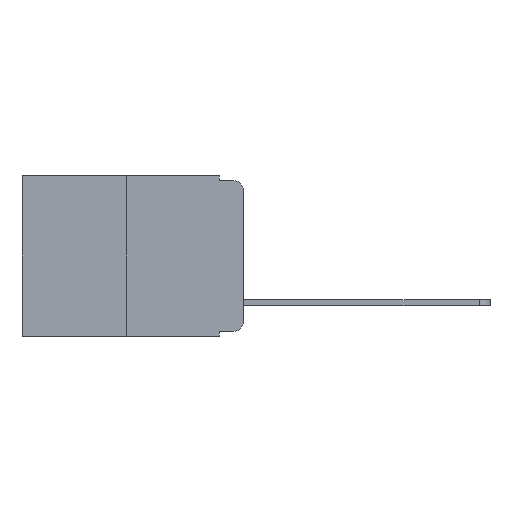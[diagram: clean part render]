
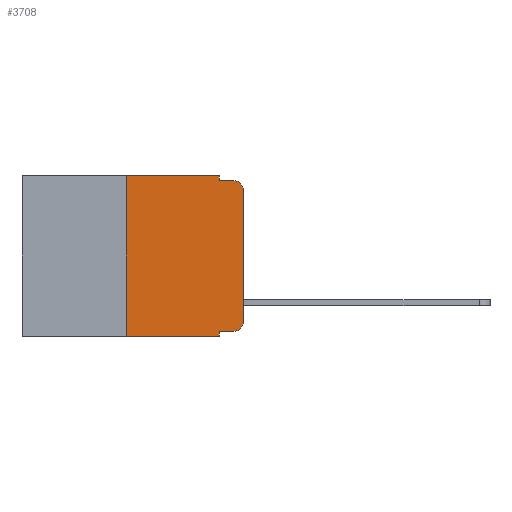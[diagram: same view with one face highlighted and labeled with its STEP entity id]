
A CAD part, left-side view. The second image highlights one B-rep face of the part: STEP entity #3708.
In plain terms, the highlighted planar face has unit normal (-1, 0, 0).
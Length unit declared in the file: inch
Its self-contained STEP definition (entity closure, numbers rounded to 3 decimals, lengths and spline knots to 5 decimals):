
#467 = ORIENTED_EDGE ( 'NONE', *, *, #6328, .F. ) ;
#604 = VERTEX_POINT ( 'NONE', #6772 ) ;
#728 = VERTEX_POINT ( 'NONE', #13608 ) ;
#889 = AXIS2_PLACEMENT_3D ( 'NONE', #8602, #965, #9829 ) ;
#965 = DIRECTION ( 'NONE',  ( -1., 0., 0. ) ) ;
#1081 = EDGE_CURVE ( 'NONE', #11808, #11613, #7560, .T. ) ;
#1479 = CARTESIAN_POINT ( 'NONE',  ( 0., 0.051, -0.01 ) ) ;
#1660 = EDGE_CURVE ( 'NONE', #11613, #728, #3568, .T. ) ;
#1695 = ORIENTED_EDGE ( 'NONE', *, *, #7569, .T. ) ;
#1840 = VERTEX_POINT ( 'NONE', #5149 ) ;
#2181 = CARTESIAN_POINT ( 'NONE',  ( 0., 0., -0.03 ) ) ;
#2254 = CARTESIAN_POINT ( 'NONE',  ( 0., 0.25, -0.343 ) ) ;
#2334 = VERTEX_POINT ( 'NONE', #11303 ) ;
#3093 = DIRECTION ( 'NONE',  ( 0., 0., -1. ) ) ;
#3274 = EDGE_CURVE ( 'NONE', #6769, #604, #13324, .T. ) ;
#3323 = AXIS2_PLACEMENT_3D ( 'NONE', #9423, #9931, #14495 ) ;
#3479 = LINE ( 'NONE', #10621, #15600 ) ;
#3517 = ORIENTED_EDGE ( 'NONE', *, *, #8271, .F. ) ;
#3568 = CIRCLE ( 'NONE', #3323, 0.02 ) ;
#3708 = ADVANCED_FACE ( 'NONE', ( #3911 ), #13899, .F. ) ;
#3768 = CARTESIAN_POINT ( 'NONE',  ( 0., 0.25, 0. ) ) ;
#3861 = CARTESIAN_POINT ( 'NONE',  ( 0., 0., -0.313 ) ) ;
#3911 = FACE_OUTER_BOUND ( 'NONE', #7472, .T. ) ;
#4689 = DIRECTION ( 'NONE',  ( 1., 0., 0. ) ) ;
#4860 = LINE ( 'NONE', #8090, #14480 ) ;
#5058 = AXIS2_PLACEMENT_3D ( 'NONE', #9745, #4689, #5153 ) ;
#5149 = CARTESIAN_POINT ( 'NONE',  ( 0., 0.051, -0.343 ) ) ;
#5153 = DIRECTION ( 'NONE',  ( 0., 0., -1. ) ) ;
#5173 = DIRECTION ( 'NONE',  ( 0., -1., 0. ) ) ;
#5663 = LINE ( 'NONE', #8107, #11774 ) ;
#5972 = CARTESIAN_POINT ( 'NONE',  ( 0., 0.051, -0.333 ) ) ;
#6021 = VERTEX_POINT ( 'NONE', #2254 ) ;
#6328 = EDGE_CURVE ( 'NONE', #6021, #9548, #15046, .T. ) ;
#6550 = ORIENTED_EDGE ( 'NONE', *, *, #7190, .F. ) ;
#6769 = VERTEX_POINT ( 'NONE', #5972 ) ;
#6772 = CARTESIAN_POINT ( 'NONE',  ( 0., 0.02, -0.333 ) ) ;
#7190 = EDGE_CURVE ( 'NONE', #12098, #728, #7608, .T. ) ;
#7197 = VECTOR ( 'NONE', #8871, 39.37008 ) ;
#7472 = EDGE_LOOP ( 'NONE', ( #15298, #15630, #6550, #16004, #3517, #467, #10571, #10932, #14356, #1695 ) ) ;
#7560 = LINE ( 'NONE', #9074, #7197 ) ;
#7569 = EDGE_CURVE ( 'NONE', #604, #11808, #10555, .T. ) ;
#7608 = LINE ( 'NONE', #1479, #7998 ) ;
#7880 = DIRECTION ( 'NONE',  ( 0., -1., 0. ) ) ;
#7995 = EDGE_CURVE ( 'NONE', #2334, #12098, #3479, .T. ) ;
#7998 = VECTOR ( 'NONE', #7880, 39.37008 ) ;
#8090 = CARTESIAN_POINT ( 'NONE',  ( 0., 0.051, 0. ) ) ;
#8107 = CARTESIAN_POINT ( 'NONE',  ( 0., 0.473, -0.343 ) ) ;
#8161 = DIRECTION ( 'NONE',  ( 0., -1., 0. ) ) ;
#8271 = EDGE_CURVE ( 'NONE', #9548, #2334, #9200, .T. ) ;
#8310 = CARTESIAN_POINT ( 'NONE',  ( 0., 0.051, -0.01 ) ) ;
#8602 = CARTESIAN_POINT ( 'NONE',  ( 0., 0.02, -0.313 ) ) ;
#8871 = DIRECTION ( 'NONE',  ( 0., 0., 1. ) ) ;
#9074 = CARTESIAN_POINT ( 'NONE',  ( 0., 0., 0. ) ) ;
#9200 = LINE ( 'NONE', #11110, #15433 ) ;
#9207 = EDGE_CURVE ( 'NONE', #6769, #1840, #4860, .T. ) ;
#9423 = CARTESIAN_POINT ( 'NONE',  ( 0., 0.02, -0.03 ) ) ;
#9548 = VERTEX_POINT ( 'NONE', #3768 ) ;
#9745 = CARTESIAN_POINT ( 'NONE',  ( 0., 0.473, 0. ) ) ;
#9829 = DIRECTION ( 'NONE',  ( 0., 0., -1. ) ) ;
#9931 = DIRECTION ( 'NONE',  ( -1., 0., 0. ) ) ;
#10211 = VECTOR ( 'NONE', #5173, 39.37008 ) ;
#10555 = CIRCLE ( 'NONE', #889, 0.02 ) ;
#10571 = ORIENTED_EDGE ( 'NONE', *, *, #14046, .T. ) ;
#10621 = CARTESIAN_POINT ( 'NONE',  ( 0., 0.051, 0. ) ) ;
#10932 = ORIENTED_EDGE ( 'NONE', *, *, #9207, .F. ) ;
#11110 = CARTESIAN_POINT ( 'NONE',  ( 0., 0.473, 0. ) ) ;
#11303 = CARTESIAN_POINT ( 'NONE',  ( 0., 0.051, 0. ) ) ;
#11613 = VERTEX_POINT ( 'NONE', #2181 ) ;
#11774 = VECTOR ( 'NONE', #8161, 39.37008 ) ;
#11808 = VERTEX_POINT ( 'NONE', #3861 ) ;
#12098 = VERTEX_POINT ( 'NONE', #8310 ) ;
#12296 = DIRECTION ( 'NONE',  ( 0., -1., 0. ) ) ;
#12690 = VECTOR ( 'NONE', #15662, 39.37008 ) ;
#13324 = LINE ( 'NONE', #13895, #10211 ) ;
#13608 = CARTESIAN_POINT ( 'NONE',  ( 0., 0.02, -0.01 ) ) ;
#13895 = CARTESIAN_POINT ( 'NONE',  ( 0., 0.051, -0.333 ) ) ;
#13899 = PLANE ( 'NONE',  #5058 ) ;
#14046 = EDGE_CURVE ( 'NONE', #6021, #1840, #5663, .T. ) ;
#14356 = ORIENTED_EDGE ( 'NONE', *, *, #3274, .T. ) ;
#14480 = VECTOR ( 'NONE', #15154, 39.37008 ) ;
#14495 = DIRECTION ( 'NONE',  ( 0., 0., -1. ) ) ;
#15046 = LINE ( 'NONE', #15783, #12690 ) ;
#15154 = DIRECTION ( 'NONE',  ( 0., 0., -1. ) ) ;
#15298 = ORIENTED_EDGE ( 'NONE', *, *, #1081, .T. ) ;
#15433 = VECTOR ( 'NONE', #12296, 39.37008 ) ;
#15600 = VECTOR ( 'NONE', #3093, 39.37008 ) ;
#15630 = ORIENTED_EDGE ( 'NONE', *, *, #1660, .T. ) ;
#15662 = DIRECTION ( 'NONE',  ( 0., 0., 1. ) ) ;
#15783 = CARTESIAN_POINT ( 'NONE',  ( 0., 0.25, 0. ) ) ;
#16004 = ORIENTED_EDGE ( 'NONE', *, *, #7995, .F. ) ;
